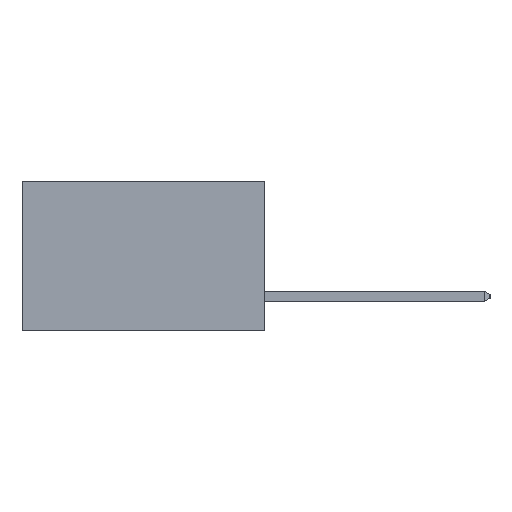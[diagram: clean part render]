
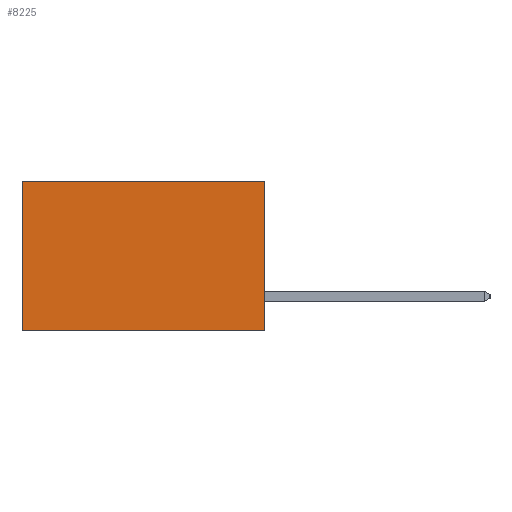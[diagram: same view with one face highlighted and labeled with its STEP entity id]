
A CAD part, left-side view. The second image highlights one B-rep face of the part: STEP entity #8225.
In plain terms, the highlighted planar face has unit normal (-1, 0, 0).
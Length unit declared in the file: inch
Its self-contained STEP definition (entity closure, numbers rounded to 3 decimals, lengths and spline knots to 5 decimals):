
#388 = CARTESIAN_POINT ( 'NONE',  ( 0.2615, 0., -0.37 ) ) ;
#774 = CARTESIAN_POINT ( 'NONE',  ( 0.2615, 0., 0. ) ) ;
#890 = VECTOR ( 'NONE', #5149, 39.37008 ) ;
#1947 = VERTEX_POINT ( 'NONE', #9458 ) ;
#1954 = DIRECTION ( 'NONE',  ( 1., 0., 0. ) ) ;
#2186 = EDGE_CURVE ( 'NONE', #3320, #9686, #13930, .T. ) ;
#2299 = ORIENTED_EDGE ( 'NONE', *, *, #18393, .T. ) ;
#2676 = DIRECTION ( 'NONE',  ( 0., 0., -1. ) ) ;
#3320 = VERTEX_POINT ( 'NONE', #9939 ) ;
#3827 = VECTOR ( 'NONE', #2676, 39.37008 ) ;
#4149 = DIRECTION ( 'NONE',  ( 0., 1., 0. ) ) ;
#5025 = PLANE ( 'NONE',  #9719 ) ;
#5037 = CARTESIAN_POINT ( 'NONE',  ( 0.2615, 0., -0.37 ) ) ;
#5149 = DIRECTION ( 'NONE',  ( 0., 1., 0. ) ) ;
#5943 = CARTESIAN_POINT ( 'NONE',  ( 0.2615, 0.6, -0.37 ) ) ;
#6233 = VERTEX_POINT ( 'NONE', #774 ) ;
#6587 = VECTOR ( 'NONE', #4149, 39.37008 ) ;
#8104 = LINE ( 'NONE', #13630, #3827 ) ;
#8225 = ADVANCED_FACE ( 'NONE', ( #10734 ), #5025, .F. ) ;
#8788 = ORIENTED_EDGE ( 'NONE', *, *, #18469, .T. ) ;
#9101 = EDGE_CURVE ( 'NONE', #6233, #3320, #8104, .T. ) ;
#9458 = CARTESIAN_POINT ( 'NONE',  ( 0.2615, 0.6, 0. ) ) ;
#9686 = VERTEX_POINT ( 'NONE', #10497 ) ;
#9719 = AXIS2_PLACEMENT_3D ( 'NONE', #388, #1954, #12982 ) ;
#9939 = CARTESIAN_POINT ( 'NONE',  ( 0.2615, 0., -0.37 ) ) ;
#10497 = CARTESIAN_POINT ( 'NONE',  ( 0.2615, 0.6, -0.37 ) ) ;
#10734 = FACE_OUTER_BOUND ( 'NONE', #14510, .T. ) ;
#11991 = VECTOR ( 'NONE', #16843, 39.37008 ) ;
#12781 = ORIENTED_EDGE ( 'NONE', *, *, #2186, .F. ) ;
#12982 = DIRECTION ( 'NONE',  ( 0., 0., -1. ) ) ;
#13630 = CARTESIAN_POINT ( 'NONE',  ( 0.2615, 0., -0.37 ) ) ;
#13930 = LINE ( 'NONE', #5037, #890 ) ;
#13952 = LINE ( 'NONE', #19683, #6587 ) ;
#13962 = ORIENTED_EDGE ( 'NONE', *, *, #9101, .F. ) ;
#14510 = EDGE_LOOP ( 'NONE', ( #8788, #12781, #13962, #2299 ) ) ;
#16843 = DIRECTION ( 'NONE',  ( 0., 0., -1. ) ) ;
#18393 = EDGE_CURVE ( 'NONE', #6233, #1947, #13952, .T. ) ;
#18469 = EDGE_CURVE ( 'NONE', #1947, #9686, #20095, .T. ) ;
#19683 = CARTESIAN_POINT ( 'NONE',  ( 0.2615, 0., 0. ) ) ;
#20095 = LINE ( 'NONE', #5943, #11991 ) ;
